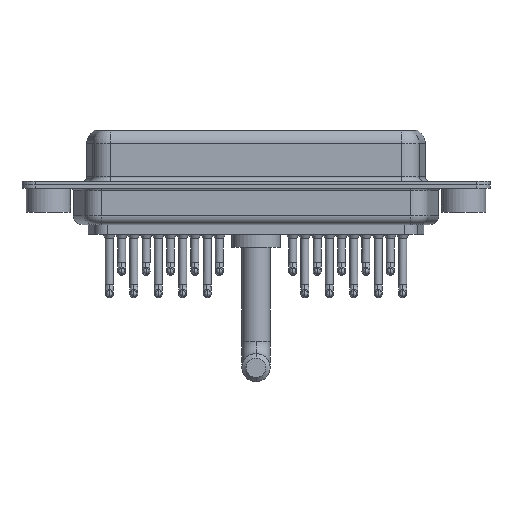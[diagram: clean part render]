
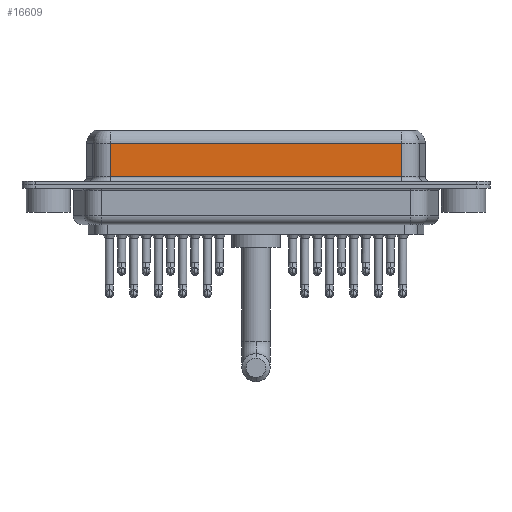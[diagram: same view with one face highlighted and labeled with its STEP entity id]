
A CAD part, front view. The second image highlights one B-rep face of the part: STEP entity #16609.
In plain terms, the highlighted planar face has unit normal (0, -1, 0).
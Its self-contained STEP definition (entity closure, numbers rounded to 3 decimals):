
#403 = CARTESIAN_POINT ( 'NONE',  ( 40.037, -3.95, 6.4 ) ) ;
#496 = LINE ( 'NONE', #611, #11896 ) ;
#611 = CARTESIAN_POINT ( 'NONE',  ( 40.037, -3.95, 6.4 ) ) ;
#2002 = DIRECTION ( 'NONE',  ( 0., 0., -1. ) ) ;
#3179 = CARTESIAN_POINT ( 'NONE',  ( 40.037, -3.95, 0.9 ) ) ;
#3406 = CARTESIAN_POINT ( 'NONE',  ( 40.037, -3.95, 4.65 ) ) ;
#3840 = VECTOR ( 'NONE', #2002, 1000. ) ;
#3878 = AXIS2_PLACEMENT_3D ( 'NONE', #403, #21406, #8794 ) ;
#5299 = VECTOR ( 'NONE', #20156, 1000. ) ;
#5794 = ORIENTED_EDGE ( 'NONE', *, *, #21405, .T. ) ;
#5893 = DIRECTION ( 'NONE',  ( 0., 0., -1. ) ) ;
#6965 = ORIENTED_EDGE ( 'NONE', *, *, #7019, .T. ) ;
#7019 = EDGE_CURVE ( 'NONE', #8264, #10713, #19146, .T. ) ;
#7502 = EDGE_LOOP ( 'NONE', ( #7628, #6965, #20538, #5794 ) ) ;
#7628 = ORIENTED_EDGE ( 'NONE', *, *, #21864, .F. ) ;
#8264 = VERTEX_POINT ( 'NONE', #13158 ) ;
#8794 = DIRECTION ( 'NONE',  ( 0., 0., 1. ) ) ;
#8911 = DIRECTION ( 'NONE',  ( -1., 0., 0. ) ) ;
#9902 = CARTESIAN_POINT ( 'NONE',  ( 7.013, -3.95, 0.9 ) ) ;
#10167 = VECTOR ( 'NONE', #8911, 1000. ) ;
#10597 = LINE ( 'NONE', #15895, #3840 ) ;
#10713 = VERTEX_POINT ( 'NONE', #13356 ) ;
#11306 = CARTESIAN_POINT ( 'NONE',  ( 40.037, -3.95, 0.9 ) ) ;
#11896 = VECTOR ( 'NONE', #5893, 1000. ) ;
#13158 = CARTESIAN_POINT ( 'NONE',  ( 40.037, -3.95, 4.65 ) ) ;
#13356 = CARTESIAN_POINT ( 'NONE',  ( 7.013, -3.95, 4.65 ) ) ;
#15186 = VERTEX_POINT ( 'NONE', #9902 ) ;
#15895 = CARTESIAN_POINT ( 'NONE',  ( 7.013, -3.95, 6.4 ) ) ;
#16609 = ADVANCED_FACE ( 'NONE', ( #17526 ), #19686, .F. ) ;
#17526 = FACE_OUTER_BOUND ( 'NONE', #7502, .T. ) ;
#18540 = LINE ( 'NONE', #11306, #5299 ) ;
#19146 = LINE ( 'NONE', #3406, #10167 ) ;
#19686 = PLANE ( 'NONE',  #3878 ) ;
#20156 = DIRECTION ( 'NONE',  ( 1., 0., 0. ) ) ;
#20538 = ORIENTED_EDGE ( 'NONE', *, *, #21742, .T. ) ;
#21023 = VERTEX_POINT ( 'NONE', #3179 ) ;
#21405 = EDGE_CURVE ( 'NONE', #15186, #21023, #18540, .T. ) ;
#21406 = DIRECTION ( 'NONE',  ( 0., 1., 0. ) ) ;
#21742 = EDGE_CURVE ( 'NONE', #10713, #15186, #10597, .T. ) ;
#21864 = EDGE_CURVE ( 'NONE', #8264, #21023, #496, .T. ) ;
